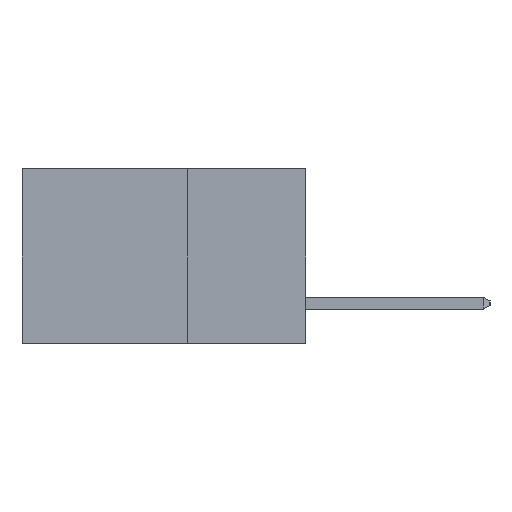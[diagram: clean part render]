
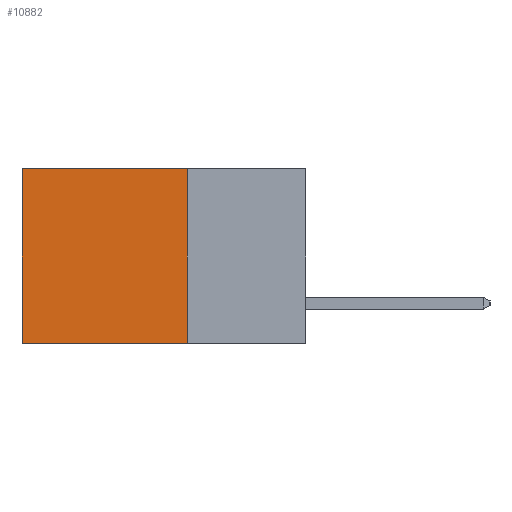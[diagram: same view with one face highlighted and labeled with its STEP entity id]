
A CAD part, left-side view. The second image highlights one B-rep face of the part: STEP entity #10882.
In plain terms, the highlighted planar face has unit normal (-1, 0, 0).
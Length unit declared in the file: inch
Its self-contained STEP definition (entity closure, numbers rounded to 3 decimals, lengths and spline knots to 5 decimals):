
#51 = ORIENTED_EDGE ( 'NONE', *, *, #8323, .T. ) ;
#400 = LINE ( 'NONE', #8581, #8399 ) ;
#627 = DIRECTION ( 'NONE',  ( 0., 0., -1. ) ) ;
#893 = DIRECTION ( 'NONE',  ( 0., 1., 0. ) ) ;
#1366 = CARTESIAN_POINT ( 'NONE',  ( 0.2615, 0.25, 0. ) ) ;
#1590 = VECTOR ( 'NONE', #8212, 39.37008 ) ;
#2406 = VECTOR ( 'NONE', #7262, 39.37008 ) ;
#2721 = EDGE_CURVE ( 'NONE', #12485, #12131, #400, .T. ) ;
#3732 = PLANE ( 'NONE',  #5861 ) ;
#5177 = ORIENTED_EDGE ( 'NONE', *, *, #10460, .T. ) ;
#5861 = AXIS2_PLACEMENT_3D ( 'NONE', #11876, #6895, #627 ) ;
#6895 = DIRECTION ( 'NONE',  ( 1., 0., 0. ) ) ;
#7223 = CARTESIAN_POINT ( 'NONE',  ( 0.2615, 0.25, -0.37 ) ) ;
#7262 = DIRECTION ( 'NONE',  ( 0., 1., 0. ) ) ;
#7525 = VERTEX_POINT ( 'NONE', #1366 ) ;
#7662 = ORIENTED_EDGE ( 'NONE', *, *, #9144, .F. ) ;
#7778 = DIRECTION ( 'NONE',  ( 0., 0., -1. ) ) ;
#8212 = DIRECTION ( 'NONE',  ( 0., 0., -1. ) ) ;
#8302 = CARTESIAN_POINT ( 'NONE',  ( 0.2615, 0.25, 0. ) ) ;
#8323 = EDGE_CURVE ( 'NONE', #11994, #12131, #9262, .T. ) ;
#8399 = VECTOR ( 'NONE', #893, 39.37008 ) ;
#8581 = CARTESIAN_POINT ( 'NONE',  ( 0.2615, 0.25, -0.37 ) ) ;
#8935 = VECTOR ( 'NONE', #7778, 39.37008 ) ;
#9144 = EDGE_CURVE ( 'NONE', #7525, #12485, #12136, .T. ) ;
#9262 = LINE ( 'NONE', #11780, #8935 ) ;
#9689 = CARTESIAN_POINT ( 'NONE',  ( 0.2615, 0.25, -0.37 ) ) ;
#10460 = EDGE_CURVE ( 'NONE', #7525, #11994, #13151, .T. ) ;
#10567 = EDGE_LOOP ( 'NONE', ( #51, #12446, #7662, #5177 ) ) ;
#10603 = FACE_OUTER_BOUND ( 'NONE', #10567, .T. ) ;
#10882 = ADVANCED_FACE ( 'NONE', ( #10603 ), #3732, .F. ) ;
#11136 = CARTESIAN_POINT ( 'NONE',  ( 0.2615, 0.6, -0.37 ) ) ;
#11682 = CARTESIAN_POINT ( 'NONE',  ( 0.2615, 0.6, 0. ) ) ;
#11780 = CARTESIAN_POINT ( 'NONE',  ( 0.2615, 0.6, -0.37 ) ) ;
#11876 = CARTESIAN_POINT ( 'NONE',  ( 0.2615, 0.25, -0.37 ) ) ;
#11994 = VERTEX_POINT ( 'NONE', #11682 ) ;
#12131 = VERTEX_POINT ( 'NONE', #11136 ) ;
#12136 = LINE ( 'NONE', #7223, #1590 ) ;
#12446 = ORIENTED_EDGE ( 'NONE', *, *, #2721, .F. ) ;
#12485 = VERTEX_POINT ( 'NONE', #9689 ) ;
#13151 = LINE ( 'NONE', #8302, #2406 ) ;
